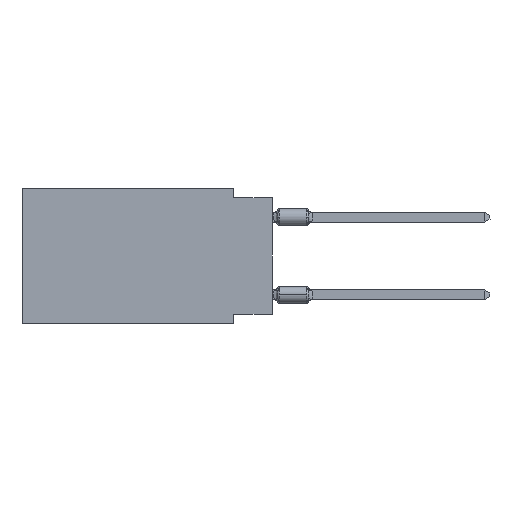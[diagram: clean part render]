
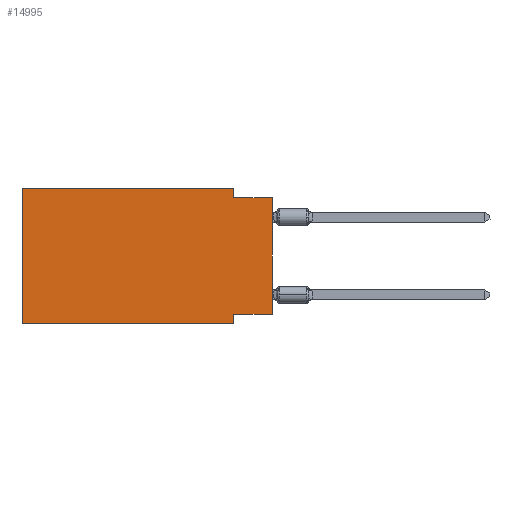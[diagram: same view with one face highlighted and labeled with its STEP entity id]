
A CAD part, left-side view. The second image highlights one B-rep face of the part: STEP entity #14995.
In plain terms, the highlighted planar face has unit normal (-1, 0, 0).
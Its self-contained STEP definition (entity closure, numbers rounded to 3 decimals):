
#1 = CARTESIAN_POINT ( 'NONE',  ( 0., 2.54, -8.89 ) ) ;
#1038 = ORIENTED_EDGE ( 'NONE', *, *, #3202, .F. ) ;
#1292 = VECTOR ( 'NONE', #14100, 1000. ) ;
#1318 = DIRECTION ( 'NONE',  ( 0., 0., -1. ) ) ;
#1340 = DIRECTION ( 'NONE',  ( 0., 1., 0. ) ) ;
#1401 = EDGE_CURVE ( 'NONE', #2906, #18761, #4298, .T. ) ;
#1797 = VERTEX_POINT ( 'NONE', #13822 ) ;
#2214 = CARTESIAN_POINT ( 'NONE',  ( 0., 2.54, -8.89 ) ) ;
#2429 = CARTESIAN_POINT ( 'NONE',  ( 0., 2.54, -0.635 ) ) ;
#2906 = VERTEX_POINT ( 'NONE', #12802 ) ;
#3202 = EDGE_CURVE ( 'NONE', #18593, #1797, #5411, .T. ) ;
#3288 = VECTOR ( 'NONE', #20842, 1000. ) ;
#4041 = ORIENTED_EDGE ( 'NONE', *, *, #20154, .F. ) ;
#4084 = CARTESIAN_POINT ( 'NONE',  ( 0., 16.383, 0. ) ) ;
#4246 = FACE_OUTER_BOUND ( 'NONE', #11248, .T. ) ;
#4298 = LINE ( 'NONE', #8907, #5670 ) ;
#4624 = LINE ( 'NONE', #20955, #9166 ) ;
#5056 = VECTOR ( 'NONE', #11943, 1000. ) ;
#5411 = LINE ( 'NONE', #20331, #5056 ) ;
#5670 = VECTOR ( 'NONE', #15565, 1000. ) ;
#5848 = ORIENTED_EDGE ( 'NONE', *, *, #1401, .F. ) ;
#5952 = DIRECTION ( 'NONE',  ( 1., 0., 0. ) ) ;
#6351 = VECTOR ( 'NONE', #21104, 1000. ) ;
#6794 = LINE ( 'NONE', #13340, #15329 ) ;
#7710 = CARTESIAN_POINT ( 'NONE',  ( 0., 0., 0. ) ) ;
#7857 = CARTESIAN_POINT ( 'NONE',  ( 0., 0., -8.255 ) ) ;
#8907 = CARTESIAN_POINT ( 'NONE',  ( 0., 16.383, 0. ) ) ;
#9045 = EDGE_CURVE ( 'NONE', #11921, #20712, #20254, .T. ) ;
#9166 = VECTOR ( 'NONE', #1318, 1000. ) ;
#9256 = CARTESIAN_POINT ( 'NONE',  ( 0., 16.383, 0. ) ) ;
#9322 = LINE ( 'NONE', #7710, #3288 ) ;
#9331 = ORIENTED_EDGE ( 'NONE', *, *, #17339, .F. ) ;
#9599 = CARTESIAN_POINT ( 'NONE',  ( 0., 16.383, 0. ) ) ;
#10369 = EDGE_CURVE ( 'NONE', #2906, #20712, #6794, .T. ) ;
#10435 = CARTESIAN_POINT ( 'NONE',  ( 0., 0., -8.255 ) ) ;
#11248 = EDGE_LOOP ( 'NONE', ( #12194, #1038, #4041, #9331, #5848, #15259, #20083, #14514 ) ) ;
#11921 = VERTEX_POINT ( 'NONE', #16736 ) ;
#11943 = DIRECTION ( 'NONE',  ( 0., -1., 0. ) ) ;
#12194 = ORIENTED_EDGE ( 'NONE', *, *, #16947, .T. ) ;
#12237 = VECTOR ( 'NONE', #1340, 1000. ) ;
#12497 = DIRECTION ( 'NONE',  ( 0., 0., -1. ) ) ;
#12502 = AXIS2_PLACEMENT_3D ( 'NONE', #9599, #5952, #12497 ) ;
#12802 = CARTESIAN_POINT ( 'NONE',  ( 0., 16.383, -8.89 ) ) ;
#12903 = LINE ( 'NONE', #7857, #12237 ) ;
#13340 = CARTESIAN_POINT ( 'NONE',  ( 0., 16.383, -8.89 ) ) ;
#13822 = CARTESIAN_POINT ( 'NONE',  ( 0., 0., -0.635 ) ) ;
#14100 = DIRECTION ( 'NONE',  ( 0., 0., -1. ) ) ;
#14514 = ORIENTED_EDGE ( 'NONE', *, *, #18654, .F. ) ;
#14995 = ADVANCED_FACE ( 'NONE', ( #4246 ), #16043, .F. ) ;
#15146 = DIRECTION ( 'NONE',  ( 0., -1., 0. ) ) ;
#15259 = ORIENTED_EDGE ( 'NONE', *, *, #10369, .T. ) ;
#15329 = VECTOR ( 'NONE', #15146, 1000. ) ;
#15565 = DIRECTION ( 'NONE',  ( 0., 0., 1. ) ) ;
#15849 = LINE ( 'NONE', #4084, #6351 ) ;
#16043 = PLANE ( 'NONE',  #12502 ) ;
#16629 = VERTEX_POINT ( 'NONE', #19904 ) ;
#16736 = CARTESIAN_POINT ( 'NONE',  ( 0., 2.54, -8.255 ) ) ;
#16947 = EDGE_CURVE ( 'NONE', #20036, #1797, #9322, .T. ) ;
#17339 = EDGE_CURVE ( 'NONE', #18761, #16629, #15849, .T. ) ;
#18593 = VERTEX_POINT ( 'NONE', #2429 ) ;
#18654 = EDGE_CURVE ( 'NONE', #20036, #11921, #12903, .T. ) ;
#18761 = VERTEX_POINT ( 'NONE', #9256 ) ;
#19904 = CARTESIAN_POINT ( 'NONE',  ( 0., 2.54, 0. ) ) ;
#20036 = VERTEX_POINT ( 'NONE', #10435 ) ;
#20083 = ORIENTED_EDGE ( 'NONE', *, *, #9045, .F. ) ;
#20154 = EDGE_CURVE ( 'NONE', #16629, #18593, #4624, .T. ) ;
#20254 = LINE ( 'NONE', #2214, #1292 ) ;
#20331 = CARTESIAN_POINT ( 'NONE',  ( 0., 0., -0.635 ) ) ;
#20712 = VERTEX_POINT ( 'NONE', #1 ) ;
#20842 = DIRECTION ( 'NONE',  ( 0., 0., 1. ) ) ;
#20955 = CARTESIAN_POINT ( 'NONE',  ( 0., 2.54, 0. ) ) ;
#21104 = DIRECTION ( 'NONE',  ( 0., -1., 0. ) ) ;
